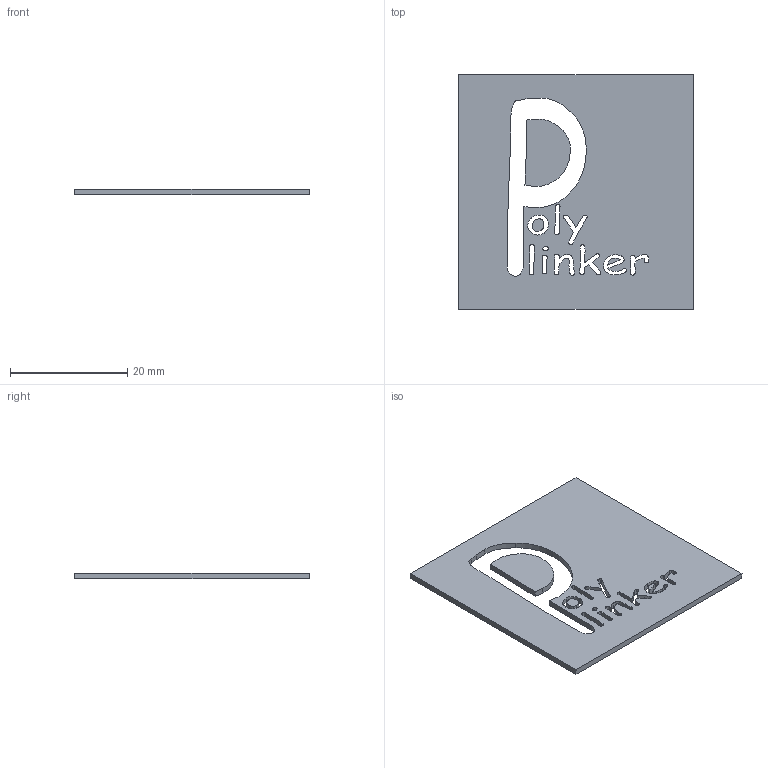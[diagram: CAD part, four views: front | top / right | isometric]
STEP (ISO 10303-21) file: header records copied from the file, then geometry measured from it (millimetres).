
FILE_DESCRIPTION (( 'STEP AP214' ), '1' );
FILE_NAME ('PolyPlinkerTile.step', '2019-12-18T03:08:27', ( '' ), ( '' ), 'SwSTEP 2.0', 'SolidWorks 2019', '' );
FILE_SCHEMA (( 'AUTOMOTIVE_DESIGN' ));
Length unit declared in the file: millimetre
Products named in the file (1): PolyPlinkerTile
Bounding box: 40 x 40 x 1 mm (x, y, z)
Volume: 1384.4 mm3; surface area: 3182.2 mm2
Topology: 4 solids, 4 shells, 231 faces, 669 edges, 446 vertices
Faces by surface type: bspline 194, plane 37
Entity records: 8712 total; most frequent: CARTESIAN_POINT 3869, ORIENTED_EDGE 1338, EDGE_CURVE 669, VERTEX_POINT 446, B_SPLINE_CURVE_WITH_KNOTS 388, DIRECTION 357, VECTOR 281, LINE 281
